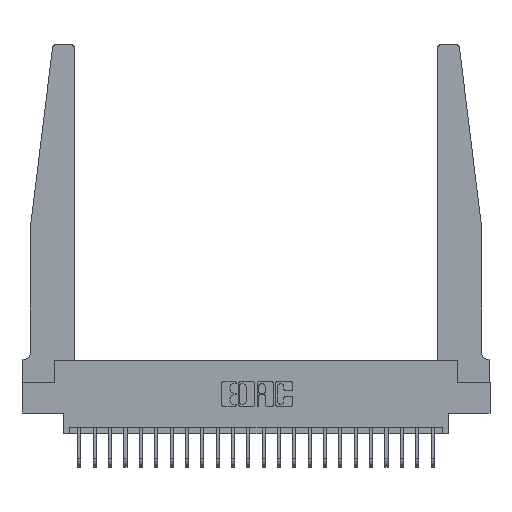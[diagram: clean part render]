
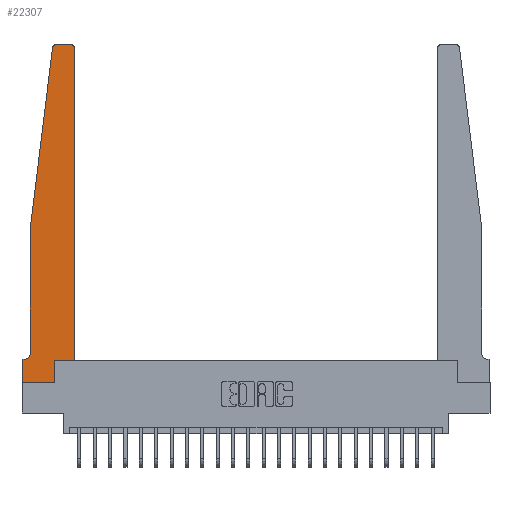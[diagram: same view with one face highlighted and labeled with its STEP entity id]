
A CAD part, top view. The second image highlights one B-rep face of the part: STEP entity #22307.
In plain terms, the highlighted planar face has unit normal (0, 0, 1).
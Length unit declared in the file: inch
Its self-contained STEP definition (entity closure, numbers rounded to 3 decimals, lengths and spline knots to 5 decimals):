
#59 = DIRECTION ( 'NONE',  ( -0.122, -0.992, 0. ) ) ;
#157 = DIRECTION ( 'NONE',  ( 0., 0., 1. ) ) ;
#437 = EDGE_CURVE ( 'NONE', #21443, #16322, #4945, .T. ) ;
#492 = LINE ( 'NONE', #19988, #22288 ) ;
#815 = DIRECTION ( 'NONE',  ( 1., 0., 0. ) ) ;
#945 = DIRECTION ( 'NONE',  ( 0., 1., 0. ) ) ;
#1450 = DIRECTION ( 'NONE',  ( 0., -1., 0. ) ) ;
#1477 = EDGE_CURVE ( 'NONE', #16882, #21443, #4625, .T. ) ;
#2343 = DIRECTION ( 'NONE',  ( 0., 1., 0. ) ) ;
#2381 = CARTESIAN_POINT ( 'NONE',  ( 0.395, 2.72, 0.37 ) ) ;
#2988 = LINE ( 'NONE', #15231, #7061 ) ;
#3061 = AXIS2_PLACEMENT_3D ( 'NONE', #2381, #14462, #4109 ) ;
#3544 = EDGE_CURVE ( 'NONE', #17137, #10483, #492, .T. ) ;
#3662 = DIRECTION ( 'NONE',  ( 0., 0., -1. ) ) ;
#3690 = CARTESIAN_POINT ( 'NONE',  ( 0.425, 2.72, 0.37 ) ) ;
#3726 = DIRECTION ( 'NONE',  ( -1., 0., 0. ) ) ;
#4109 = DIRECTION ( 'NONE',  ( 1., 0., 0. ) ) ;
#4321 = ORIENTED_EDGE ( 'NONE', *, *, #8314, .T. ) ;
#4328 = CIRCLE ( 'NONE', #10142, 0.03 ) ;
#4605 = CARTESIAN_POINT ( 'NONE',  ( 0.2605, 0., 0.37 ) ) ;
#4625 = LINE ( 'NONE', #10664, #13293 ) ;
#4697 = LINE ( 'NONE', #14420, #17921 ) ;
#4945 = LINE ( 'NONE', #9579, #11177 ) ;
#5309 = LINE ( 'NONE', #10088, #13427 ) ;
#6025 = VERTEX_POINT ( 'NONE', #17829 ) ;
#6597 = EDGE_CURVE ( 'NONE', #16440, #15137, #4697, .T. ) ;
#6844 = VECTOR ( 'NONE', #59, 39.37008 ) ;
#7061 = VECTOR ( 'NONE', #16884, 39.37008 ) ;
#7535 = EDGE_CURVE ( 'NONE', #11190, #21460, #18934, .T. ) ;
#7675 = AXIS2_PLACEMENT_3D ( 'NONE', #14560, #11175, #815 ) ;
#8314 = EDGE_CURVE ( 'NONE', #15137, #6025, #19313, .T. ) ;
#8589 = EDGE_CURVE ( 'NONE', #21460, #16882, #5309, .T. ) ;
#8879 = VERTEX_POINT ( 'NONE', #16027 ) ;
#9269 = VECTOR ( 'NONE', #3726, 39.37008 ) ;
#9579 = CARTESIAN_POINT ( 'NONE',  ( 0.2605, 0.18, 0.37 ) ) ;
#9694 = CIRCLE ( 'NONE', #15955, 0.05 ) ;
#10088 = CARTESIAN_POINT ( 'NONE',  ( 0., 0., 0.37 ) ) ;
#10142 = AXIS2_PLACEMENT_3D ( 'NONE', #10551, #157, #12283 ) ;
#10444 = ORIENTED_EDGE ( 'NONE', *, *, #437, .T. ) ;
#10483 = VERTEX_POINT ( 'NONE', #20723 ) ;
#10551 = CARTESIAN_POINT ( 'NONE',  ( 0.27653, 2.72, 0.37 ) ) ;
#10664 = CARTESIAN_POINT ( 'NONE',  ( 0., 0., 0.37 ) ) ;
#11175 = DIRECTION ( 'NONE',  ( 0., 0., 1. ) ) ;
#11177 = VECTOR ( 'NONE', #945, 39.37008 ) ;
#11190 = VERTEX_POINT ( 'NONE', #14536 ) ;
#11352 = CARTESIAN_POINT ( 'NONE',  ( 0., 0., 0.37 ) ) ;
#11435 = DIRECTION ( 'NONE',  ( 0., -1., 0. ) ) ;
#11437 = CARTESIAN_POINT ( 'NONE',  ( 0.425, 0.18, 0.37 ) ) ;
#11568 = ORIENTED_EDGE ( 'NONE', *, *, #11618, .T. ) ;
#11618 = EDGE_CURVE ( 'NONE', #8879, #17137, #19482, .T. ) ;
#11636 = ORIENTED_EDGE ( 'NONE', *, *, #8589, .T. ) ;
#11744 = CARTESIAN_POINT ( 'NONE',  ( 0.27653, 2.75, 0.37 ) ) ;
#11815 = ORIENTED_EDGE ( 'NONE', *, *, #6597, .T. ) ;
#12197 = CARTESIAN_POINT ( 'NONE',  ( 0.065, 1.25, 0.37 ) ) ;
#12283 = DIRECTION ( 'NONE',  ( 1., 0., 0. ) ) ;
#12322 = ORIENTED_EDGE ( 'NONE', *, *, #15815, .T. ) ;
#12352 = CARTESIAN_POINT ( 'NONE',  ( 0.065, 0.1875, 0.37 ) ) ;
#12694 = FACE_OUTER_BOUND ( 'NONE', #21445, .T. ) ;
#12723 = ORIENTED_EDGE ( 'NONE', *, *, #12920, .T. ) ;
#12744 = EDGE_CURVE ( 'NONE', #16322, #16440, #2988, .T. ) ;
#12890 = CARTESIAN_POINT ( 'NONE',  ( 0.2605, 0.18, 0.37 ) ) ;
#12920 = EDGE_CURVE ( 'NONE', #18200, #8879, #4328, .T. ) ;
#13293 = VECTOR ( 'NONE', #14121, 39.37008 ) ;
#13427 = VECTOR ( 'NONE', #1450, 39.37008 ) ;
#13599 = ORIENTED_EDGE ( 'NONE', *, *, #12744, .T. ) ;
#14019 = CARTESIAN_POINT ( 'NONE',  ( 0.015, 0.2375, 0.37 ) ) ;
#14121 = DIRECTION ( 'NONE',  ( 1., 0., 0. ) ) ;
#14420 = CARTESIAN_POINT ( 'NONE',  ( 0.425, 0.18, 0.37 ) ) ;
#14462 = DIRECTION ( 'NONE',  ( 0., 0., 1. ) ) ;
#14536 = CARTESIAN_POINT ( 'NONE',  ( 0.015, 0.1875, 0.37 ) ) ;
#14560 = CARTESIAN_POINT ( 'NONE',  ( 0., 0.1875, 0.37 ) ) ;
#14916 = ORIENTED_EDGE ( 'NONE', *, *, #1477, .T. ) ;
#15137 = VERTEX_POINT ( 'NONE', #3690 ) ;
#15231 = CARTESIAN_POINT ( 'NONE',  ( 0.425, 0.18, 0.37 ) ) ;
#15747 = DIRECTION ( 'NONE',  ( -1., 0., 0. ) ) ;
#15815 = EDGE_CURVE ( 'NONE', #10483, #11190, #9694, .T. ) ;
#15955 = AXIS2_PLACEMENT_3D ( 'NONE', #14019, #3662, #15747 ) ;
#16027 = CARTESIAN_POINT ( 'NONE',  ( 0.24675, 2.72367, 0.37 ) ) ;
#16057 = DIRECTION ( 'NONE',  ( -1., 0., 0. ) ) ;
#16322 = VERTEX_POINT ( 'NONE', #12890 ) ;
#16440 = VERTEX_POINT ( 'NONE', #11437 ) ;
#16882 = VERTEX_POINT ( 'NONE', #11352 ) ;
#16884 = DIRECTION ( 'NONE',  ( 1., 0., 0. ) ) ;
#17137 = VERTEX_POINT ( 'NONE', #22252 ) ;
#17829 = CARTESIAN_POINT ( 'NONE',  ( 0.395, 2.75, 0.37 ) ) ;
#17921 = VECTOR ( 'NONE', #2343, 39.37008 ) ;
#17944 = EDGE_CURVE ( 'NONE', #6025, #18200, #18706, .T. ) ;
#18187 = VECTOR ( 'NONE', #16057, 39.37008 ) ;
#18200 = VERTEX_POINT ( 'NONE', #11744 ) ;
#18706 = LINE ( 'NONE', #21128, #18187 ) ;
#18934 = LINE ( 'NONE', #12352, #9269 ) ;
#19246 = ORIENTED_EDGE ( 'NONE', *, *, #17944, .T. ) ;
#19313 = CIRCLE ( 'NONE', #3061, 0.03 ) ;
#19482 = LINE ( 'NONE', #12197, #6844 ) ;
#19988 = CARTESIAN_POINT ( 'NONE',  ( 0.065, 1.25, 0.37 ) ) ;
#20112 = CARTESIAN_POINT ( 'NONE',  ( 0., 0.1875, 0.37 ) ) ;
#20723 = CARTESIAN_POINT ( 'NONE',  ( 0.065, 0.2375, 0.37 ) ) ;
#21128 = CARTESIAN_POINT ( 'NONE',  ( 0.25, 2.75, 0.37 ) ) ;
#21443 = VERTEX_POINT ( 'NONE', #4605 ) ;
#21445 = EDGE_LOOP ( 'NONE', ( #19246, #12723, #11568, #22243, #12322, #21582, #11636, #14916, #10444, #13599, #11815, #4321 ) ) ;
#21446 = PLANE ( 'NONE',  #7675 ) ;
#21460 = VERTEX_POINT ( 'NONE', #20112 ) ;
#21582 = ORIENTED_EDGE ( 'NONE', *, *, #7535, .T. ) ;
#22243 = ORIENTED_EDGE ( 'NONE', *, *, #3544, .T. ) ;
#22252 = CARTESIAN_POINT ( 'NONE',  ( 0.065, 1.25, 0.37 ) ) ;
#22288 = VECTOR ( 'NONE', #11435, 39.37008 ) ;
#22307 = ADVANCED_FACE ( 'NONE', ( #12694 ), #21446, .T. ) ;
